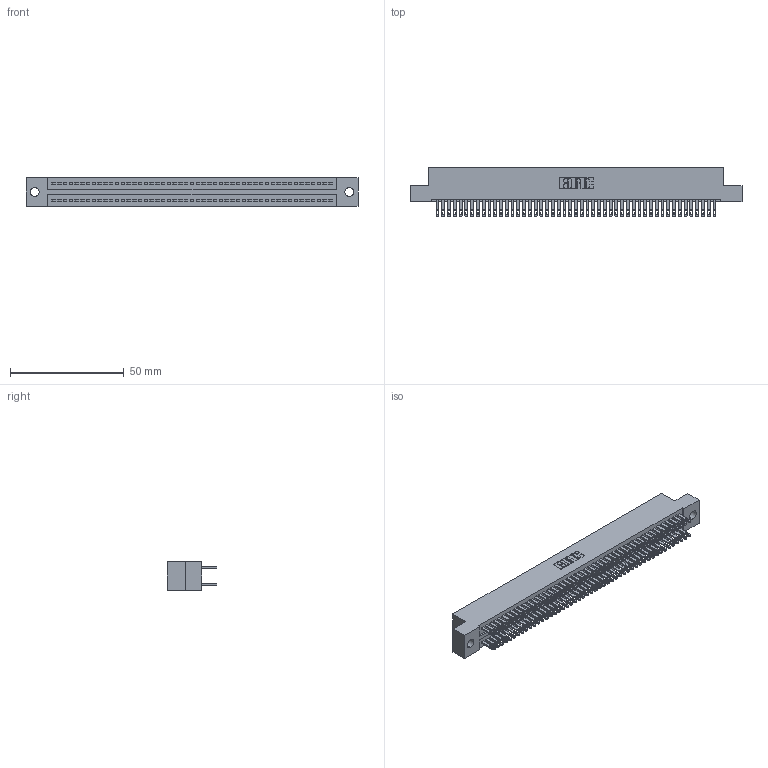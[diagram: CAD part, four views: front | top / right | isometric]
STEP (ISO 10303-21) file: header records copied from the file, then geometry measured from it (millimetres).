
FILE_DESCRIPTION (( 'STEP AP203' ), '1' );
FILE_NAME ('325-098-500-209.STEP', '2020-02-25T06:23:28', ( '' ), ( '' ), 'SwSTEP 2.0', 'SolidWorks 2016', '' );
FILE_SCHEMA (( 'CONFIG_CONTROL_DESIGN' ));
Length unit declared in the file: inch
Products named in the file (3): 325 Part_.160 TH; 325-292-001_325-293-100; 325-098-500-209
Assembly tree (99 placements, depth 2):
  325-098-500-209
    325 Part_.160 TH
    325-292-001_325-293-100  x98
Bounding box: 146.18 x 21.84 x 12.45 mm (x, y, z)
Volume: 19002.3 mm3; surface area: 24110.9 mm2
Topology: 99 solids, 99 shells, 4818 faces, 14717 edges, 9810 vertices
Faces by surface type: plane 3010, cylinder 1808
Entity records: 30551 total; most frequent: CARTESIAN_POINT 5054, ORIENTED_EDGE 4990, DIRECTION 4307, EDGE_CURVE 2495, VECTOR 2363, LINE 2363, VERTEX_POINT 1662, AXIS2_PLACEMENT_3D 972
